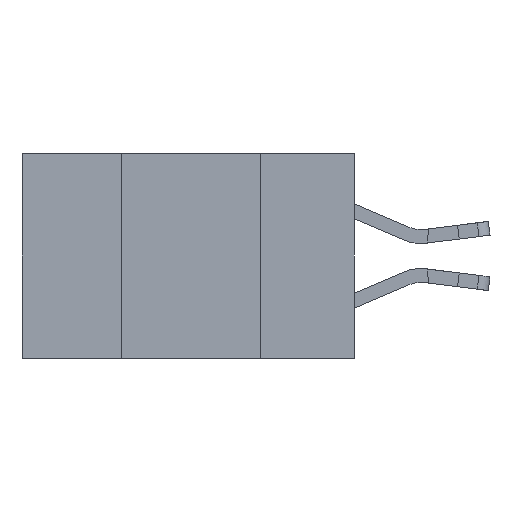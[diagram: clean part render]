
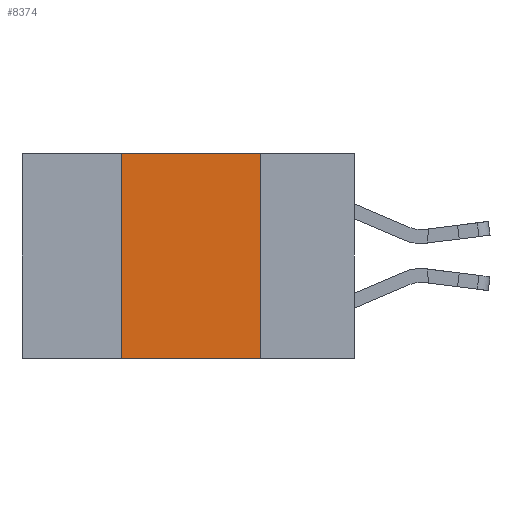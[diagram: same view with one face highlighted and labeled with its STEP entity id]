
A CAD part, left-side view. The second image highlights one B-rep face of the part: STEP entity #8374.
In plain terms, the highlighted planar face has unit normal (-1, 0, 0).
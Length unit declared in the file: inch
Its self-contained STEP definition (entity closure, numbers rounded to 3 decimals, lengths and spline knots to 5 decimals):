
#537 = DIRECTION ( 'NONE',  ( 0., -1., 0. ) ) ;
#572 = CARTESIAN_POINT ( 'NONE',  ( 0., 0.17, -0.37 ) ) ;
#1705 = CARTESIAN_POINT ( 'NONE',  ( 0., 0.42, -0.37 ) ) ;
#1987 = VERTEX_POINT ( 'NONE', #572 ) ;
#2056 = AXIS2_PLACEMENT_3D ( 'NONE', #14207, #4905, #12104 ) ;
#2216 = ORIENTED_EDGE ( 'NONE', *, *, #5190, .F. ) ;
#2445 = EDGE_CURVE ( 'NONE', #10868, #9341, #6748, .T. ) ;
#3713 = VECTOR ( 'NONE', #7473, 39.37008 ) ;
#4661 = VECTOR ( 'NONE', #6678, 39.37008 ) ;
#4739 = FACE_OUTER_BOUND ( 'NONE', #8895, .T. ) ;
#4905 = DIRECTION ( 'NONE',  ( 1., 0., 0. ) ) ;
#5190 = EDGE_CURVE ( 'NONE', #9341, #1987, #12045, .T. ) ;
#5200 = LINE ( 'NONE', #13497, #6993 ) ;
#5318 = CARTESIAN_POINT ( 'NONE',  ( 0., 0.42, -0.37 ) ) ;
#5782 = EDGE_CURVE ( 'NONE', #8483, #1987, #5200, .T. ) ;
#5920 = DIRECTION ( 'NONE',  ( 0., 0., -1. ) ) ;
#6242 = LINE ( 'NONE', #5318, #3713 ) ;
#6678 = DIRECTION ( 'NONE',  ( 0., -1., 0. ) ) ;
#6748 = LINE ( 'NONE', #13510, #4661 ) ;
#6993 = VECTOR ( 'NONE', #537, 39.37008 ) ;
#7224 = VECTOR ( 'NONE', #5920, 39.37008 ) ;
#7473 = DIRECTION ( 'NONE',  ( 0., 0., 1. ) ) ;
#8374 = ADVANCED_FACE ( 'NONE', ( #4739 ), #10941, .F. ) ;
#8461 = CARTESIAN_POINT ( 'NONE',  ( 0., 0.17, -0.37 ) ) ;
#8483 = VERTEX_POINT ( 'NONE', #1705 ) ;
#8895 = EDGE_LOOP ( 'NONE', ( #2216, #15064, #11454, #11814 ) ) ;
#9108 = CARTESIAN_POINT ( 'NONE',  ( 0., 0.42, 0. ) ) ;
#9341 = VERTEX_POINT ( 'NONE', #14795 ) ;
#9823 = EDGE_CURVE ( 'NONE', #8483, #10868, #6242, .T. ) ;
#10868 = VERTEX_POINT ( 'NONE', #9108 ) ;
#10941 = PLANE ( 'NONE',  #2056 ) ;
#11454 = ORIENTED_EDGE ( 'NONE', *, *, #9823, .F. ) ;
#11814 = ORIENTED_EDGE ( 'NONE', *, *, #5782, .T. ) ;
#12045 = LINE ( 'NONE', #8461, #7224 ) ;
#12104 = DIRECTION ( 'NONE',  ( 0., 0., -1. ) ) ;
#13497 = CARTESIAN_POINT ( 'NONE',  ( 0., 0.6, -0.37 ) ) ;
#13510 = CARTESIAN_POINT ( 'NONE',  ( 0., 0.6, 0. ) ) ;
#14207 = CARTESIAN_POINT ( 'NONE',  ( 0., 0.6, 0. ) ) ;
#14795 = CARTESIAN_POINT ( 'NONE',  ( 0., 0.17, 0. ) ) ;
#15064 = ORIENTED_EDGE ( 'NONE', *, *, #2445, .F. ) ;
